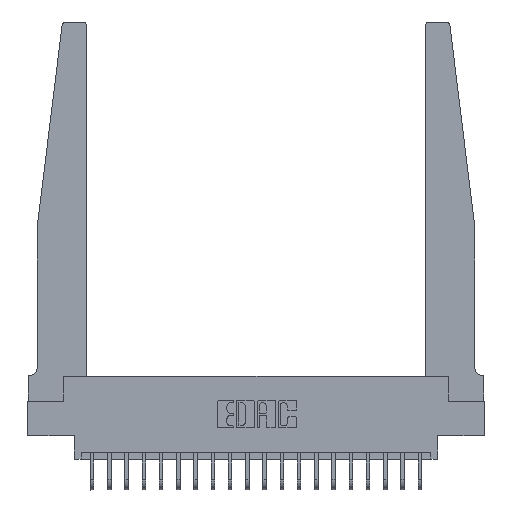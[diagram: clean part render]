
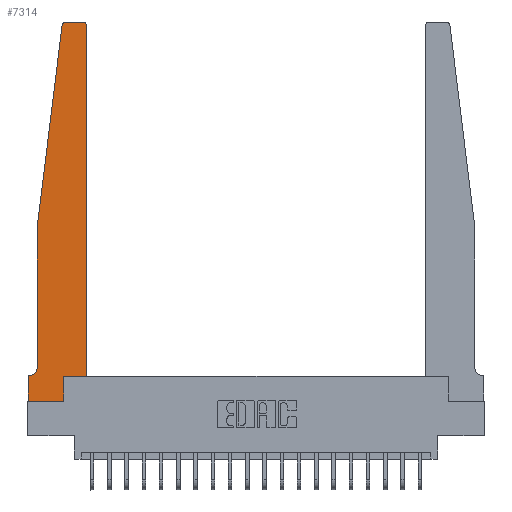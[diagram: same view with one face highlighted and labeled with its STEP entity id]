
A CAD part, top view. The second image highlights one B-rep face of the part: STEP entity #7314.
In plain terms, the highlighted planar face has unit normal (0, 0, 1).
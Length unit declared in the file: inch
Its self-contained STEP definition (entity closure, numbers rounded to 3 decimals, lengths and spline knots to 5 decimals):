
#156 = ORIENTED_EDGE ( 'NONE', *, *, #5930, .T. ) ;
#560 = CARTESIAN_POINT ( 'NONE',  ( 0.425, 0.18, 0.37 ) ) ;
#639 = LINE ( 'NONE', #7245, #3116 ) ;
#844 = DIRECTION ( 'NONE',  ( 1., 0., 0. ) ) ;
#1147 = EDGE_CURVE ( 'NONE', #18143, #21330, #3355, .T. ) ;
#1172 = DIRECTION ( 'NONE',  ( 1., 0., 0. ) ) ;
#1193 = DIRECTION ( 'NONE',  ( -0.122, -0.992, 0. ) ) ;
#1620 = ORIENTED_EDGE ( 'NONE', *, *, #6116, .T. ) ;
#2298 = LINE ( 'NONE', #16759, #4518 ) ;
#2786 = VERTEX_POINT ( 'NONE', #6134 ) ;
#3116 = VECTOR ( 'NONE', #7166, 39.37008 ) ;
#3229 = ORIENTED_EDGE ( 'NONE', *, *, #18399, .T. ) ;
#3355 = LINE ( 'NONE', #14566, #21467 ) ;
#3409 = EDGE_CURVE ( 'NONE', #11468, #22634, #18930, .T. ) ;
#3837 = ORIENTED_EDGE ( 'NONE', *, *, #1147, .T. ) ;
#4335 = EDGE_CURVE ( 'NONE', #10099, #18143, #16968, .T. ) ;
#4518 = VECTOR ( 'NONE', #844, 39.37008 ) ;
#4784 = CARTESIAN_POINT ( 'NONE',  ( 0.395, 2.72, 0.37 ) ) ;
#5296 = CARTESIAN_POINT ( 'NONE',  ( 0., 0., 0.37 ) ) ;
#5393 = DIRECTION ( 'NONE',  ( 0., 0., 1. ) ) ;
#5482 = CARTESIAN_POINT ( 'NONE',  ( 0.065, 1.25, 0.37 ) ) ;
#5874 = LINE ( 'NONE', #9982, #7789 ) ;
#5893 = DIRECTION ( 'NONE',  ( -1., 0., 0. ) ) ;
#5930 = EDGE_CURVE ( 'NONE', #19596, #2786, #639, .T. ) ;
#6079 = ORIENTED_EDGE ( 'NONE', *, *, #10476, .T. ) ;
#6116 = EDGE_CURVE ( 'NONE', #20422, #20160, #15741, .T. ) ;
#6134 = CARTESIAN_POINT ( 'NONE',  ( 0.2605, 0.18, 0.37 ) ) ;
#6668 = CARTESIAN_POINT ( 'NONE',  ( 0.065, 1.25, 0.37 ) ) ;
#7166 = DIRECTION ( 'NONE',  ( 0., 1., 0. ) ) ;
#7245 = CARTESIAN_POINT ( 'NONE',  ( 0.2605, 0.18, 0.37 ) ) ;
#7258 = VERTEX_POINT ( 'NONE', #560 ) ;
#7302 = DIRECTION ( 'NONE',  ( 0., 0., 1. ) ) ;
#7314 = ADVANCED_FACE ( 'NONE', ( #12185 ), #8881, .T. ) ;
#7369 = CARTESIAN_POINT ( 'NONE',  ( 0.065, 1.25, 0.37 ) ) ;
#7734 = CARTESIAN_POINT ( 'NONE',  ( 0.425, 0.18, 0.37 ) ) ;
#7789 = VECTOR ( 'NONE', #1172, 39.37008 ) ;
#8656 = CARTESIAN_POINT ( 'NONE',  ( 0.395, 2.75, 0.37 ) ) ;
#8745 = LINE ( 'NONE', #5296, #20233 ) ;
#8778 = AXIS2_PLACEMENT_3D ( 'NONE', #14272, #7302, #19545 ) ;
#8881 = PLANE ( 'NONE',  #8778 ) ;
#9982 = CARTESIAN_POINT ( 'NONE',  ( 0.425, 0.18, 0.37 ) ) ;
#10099 = VERTEX_POINT ( 'NONE', #12943 ) ;
#10142 = ORIENTED_EDGE ( 'NONE', *, *, #4335, .T. ) ;
#10185 = ORIENTED_EDGE ( 'NONE', *, *, #3409, .T. ) ;
#10359 = DIRECTION ( 'NONE',  ( 0., -1., 0. ) ) ;
#10476 = EDGE_CURVE ( 'NONE', #21330, #11182, #8745, .T. ) ;
#10901 = CIRCLE ( 'NONE', #21195, 0.03 ) ;
#11182 = VERTEX_POINT ( 'NONE', #14678 ) ;
#11468 = VERTEX_POINT ( 'NONE', #22676 ) ;
#11513 = EDGE_CURVE ( 'NONE', #17144, #11468, #10901, .T. ) ;
#12155 = ORIENTED_EDGE ( 'NONE', *, *, #22016, .T. ) ;
#12185 = FACE_OUTER_BOUND ( 'NONE', #19641, .T. ) ;
#12241 = ORIENTED_EDGE ( 'NONE', *, *, #13810, .T. ) ;
#12269 = CARTESIAN_POINT ( 'NONE',  ( 0.015, 0.2375, 0.37 ) ) ;
#12288 = AXIS2_PLACEMENT_3D ( 'NONE', #12269, #17658, #19322 ) ;
#12331 = DIRECTION ( 'NONE',  ( 1., 0., 0. ) ) ;
#12928 = CARTESIAN_POINT ( 'NONE',  ( 0.015, 0.1875, 0.37 ) ) ;
#12943 = CARTESIAN_POINT ( 'NONE',  ( 0.065, 0.2375, 0.37 ) ) ;
#13810 = EDGE_CURVE ( 'NONE', #20160, #17144, #14254, .T. ) ;
#14199 = CARTESIAN_POINT ( 'NONE',  ( 0.27653, 2.72, 0.37 ) ) ;
#14254 = LINE ( 'NONE', #16547, #22445 ) ;
#14266 = DIRECTION ( 'NONE',  ( 0., -1., 0. ) ) ;
#14272 = CARTESIAN_POINT ( 'NONE',  ( 0., 0.1875, 0.37 ) ) ;
#14301 = VECTOR ( 'NONE', #1193, 39.37008 ) ;
#14419 = ORIENTED_EDGE ( 'NONE', *, *, #11513, .T. ) ;
#14460 = AXIS2_PLACEMENT_3D ( 'NONE', #4784, #17031, #20617 ) ;
#14566 = CARTESIAN_POINT ( 'NONE',  ( 0.065, 0.1875, 0.37 ) ) ;
#14678 = CARTESIAN_POINT ( 'NONE',  ( 0., 0., 0.37 ) ) ;
#14924 = DIRECTION ( 'NONE',  ( 0., 1., 0. ) ) ;
#15353 = ORIENTED_EDGE ( 'NONE', *, *, #20410, .T. ) ;
#15741 = CIRCLE ( 'NONE', #14460, 0.03 ) ;
#16108 = DIRECTION ( 'NONE',  ( -1., 0., 0. ) ) ;
#16547 = CARTESIAN_POINT ( 'NONE',  ( 0.25, 2.75, 0.37 ) ) ;
#16679 = CARTESIAN_POINT ( 'NONE',  ( 0.425, 2.72, 0.37 ) ) ;
#16759 = CARTESIAN_POINT ( 'NONE',  ( 0., 0., 0.37 ) ) ;
#16941 = CARTESIAN_POINT ( 'NONE',  ( 0.2605, 0., 0.37 ) ) ;
#16968 = CIRCLE ( 'NONE', #12288, 0.05 ) ;
#17031 = DIRECTION ( 'NONE',  ( 0., 0., 1. ) ) ;
#17144 = VERTEX_POINT ( 'NONE', #21722 ) ;
#17658 = DIRECTION ( 'NONE',  ( 0., 0., -1. ) ) ;
#17973 = VECTOR ( 'NONE', #14266, 39.37008 ) ;
#18143 = VERTEX_POINT ( 'NONE', #12928 ) ;
#18399 = EDGE_CURVE ( 'NONE', #2786, #7258, #5874, .T. ) ;
#18930 = LINE ( 'NONE', #6668, #14301 ) ;
#19322 = DIRECTION ( 'NONE',  ( -1., 0., 0. ) ) ;
#19369 = CARTESIAN_POINT ( 'NONE',  ( 0., 0.1875, 0.37 ) ) ;
#19545 = DIRECTION ( 'NONE',  ( 1., 0., 0. ) ) ;
#19546 = VECTOR ( 'NONE', #14924, 39.37008 ) ;
#19596 = VERTEX_POINT ( 'NONE', #16941 ) ;
#19640 = EDGE_CURVE ( 'NONE', #22634, #10099, #22630, .T. ) ;
#19641 = EDGE_LOOP ( 'NONE', ( #12241, #14419, #10185, #21240, #10142, #3837, #6079, #15353, #156, #3229, #12155, #1620 ) ) ;
#20160 = VERTEX_POINT ( 'NONE', #8656 ) ;
#20233 = VECTOR ( 'NONE', #10359, 39.37008 ) ;
#20410 = EDGE_CURVE ( 'NONE', #11182, #19596, #2298, .T. ) ;
#20422 = VERTEX_POINT ( 'NONE', #16679 ) ;
#20617 = DIRECTION ( 'NONE',  ( 1., 0., 0. ) ) ;
#21195 = AXIS2_PLACEMENT_3D ( 'NONE', #14199, #5393, #12331 ) ;
#21240 = ORIENTED_EDGE ( 'NONE', *, *, #19640, .T. ) ;
#21330 = VERTEX_POINT ( 'NONE', #19369 ) ;
#21467 = VECTOR ( 'NONE', #16108, 39.37008 ) ;
#21722 = CARTESIAN_POINT ( 'NONE',  ( 0.27653, 2.75, 0.37 ) ) ;
#22016 = EDGE_CURVE ( 'NONE', #7258, #20422, #22287, .T. ) ;
#22287 = LINE ( 'NONE', #7734, #19546 ) ;
#22445 = VECTOR ( 'NONE', #5893, 39.37008 ) ;
#22630 = LINE ( 'NONE', #7369, #17973 ) ;
#22634 = VERTEX_POINT ( 'NONE', #5482 ) ;
#22676 = CARTESIAN_POINT ( 'NONE',  ( 0.24675, 2.72367, 0.37 ) ) ;
